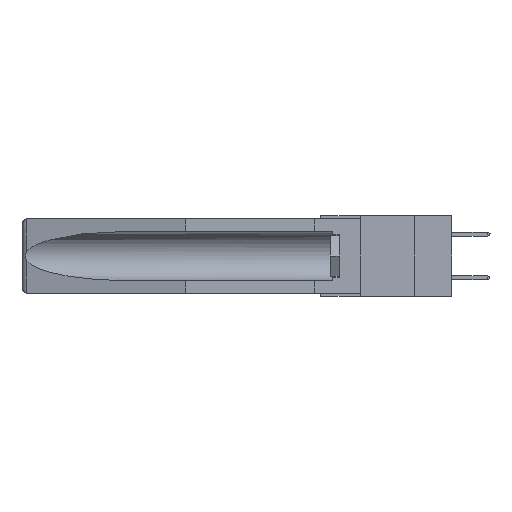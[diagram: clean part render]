
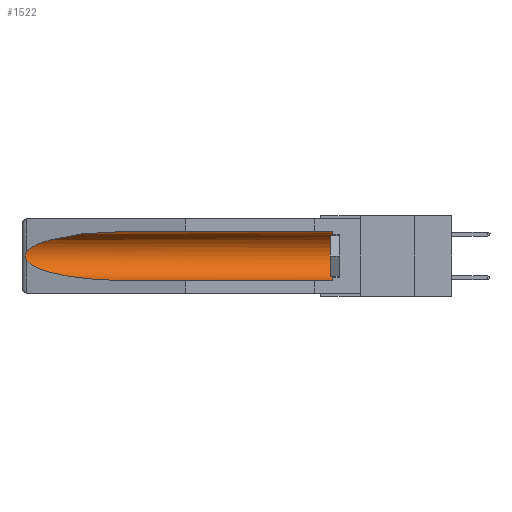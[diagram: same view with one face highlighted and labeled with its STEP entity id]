
A CAD part, left-side view. The second image highlights one B-rep face of the part: STEP entity #1522.
In plain terms, the highlighted cylindrical face has radius 2.857 mm (diameter 5.715 mm), a partial arc.
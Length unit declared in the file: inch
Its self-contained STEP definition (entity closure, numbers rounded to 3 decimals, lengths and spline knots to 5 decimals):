
#142 = ORIENTED_EDGE ( 'NONE', *, *, #10749, .T. ) ;
#1078 = VECTOR ( 'NONE', #8285, 39.37008 ) ;
#1216 = EDGE_CURVE ( 'NONE', #16953, #12645, #14009, .T. ) ;
#1220 = CARTESIAN_POINT ( 'NONE',  ( 0.155, 1.07973, -0.059 ) ) ;
#1522 = ADVANCED_FACE ( 'NONE', ( #5044 ), #20170, .F. ) ;
#1632 = AXIS2_PLACEMENT_3D ( 'NONE', #15619, #21819, #4043 ) ;
#2681 = DIRECTION ( 'NONE',  ( 0., 0., 1. ) ) ;
#3003 = CARTESIAN_POINT ( 'NONE',  ( 0.155, 0.126, -0.284 ) ) ;
#4043 = DIRECTION ( 'NONE',  ( 0., 0., 1. ) ) ;
#4476 = EDGE_CURVE ( 'NONE', #18715, #13065, #6546, .T. ) ;
#5044 = FACE_OUTER_BOUND ( 'NONE', #6459, .T. ) ;
#5306 = CARTESIAN_POINT ( 'NONE',  ( 0.26537, 1.52718, -0.19328 ) ) ;
#5474 = CARTESIAN_POINT ( 'NONE',  ( 0.26597, 1.52961, -0.15275 ) ) ;
#5706 = CARTESIAN_POINT ( 'NONE',  ( 0.155, 1.07973, -0.284 ) ) ;
#6459 = EDGE_LOOP ( 'NONE', ( #12340, #19681, #142, #18638, #24226, #20759 ) ) ;
#6535 = CARTESIAN_POINT ( 'NONE',  ( 0.25451, 1.48313, -0.24835 ) ) ;
#6546 = B_SPLINE_CURVE_WITH_KNOTS ( 'NONE', 3,
 ( #11331, #5474, #15243, #9100, #11079, #10993, #11171, #7032, #9007, #5306 ),
 .UNSPECIFIED., .F., .F.,
 ( 4, 2, 2, 2, 4 ),
 ( 0., 0.00029, 0.00058, 0.00087, 0.00117 ),
 .UNSPECIFIED. ) ;
#7032 = CARTESIAN_POINT ( 'NONE',  ( 0.26655, 1.53094, -0.18657 ) ) ;
#7169 = CARTESIAN_POINT ( 'NONE',  ( 0.26537, 1.52718, -0.14972 ) ) ;
#8103 = CARTESIAN_POINT ( 'NONE',  ( 0.26537, 1.52718, -0.19328 ) ) ;
#8140 = CARTESIAN_POINT ( 'NONE',  ( 0.155, 1.07973, -0.059 ) ) ;
#8285 = DIRECTION ( 'NONE',  ( 0., 1., 0. ) ) ;
#9007 = CARTESIAN_POINT ( 'NONE',  ( 0.26597, 1.5296, -0.19026 ) ) ;
#9100 = CARTESIAN_POINT ( 'NONE',  ( 0.2673, 1.5327, -0.16383 ) ) ;
#10027 =( BOUNDED_CURVE ( )  B_SPLINE_CURVE ( 3, ( #1220, #16964, #22873, #7169 ),
 .UNSPECIFIED., .F., .T. ) 
 B_SPLINE_CURVE_WITH_KNOTS ( ( 4, 4 ),
 ( 4.71239, 6.08839 ),
 .UNSPECIFIED. ) 
 CURVE ( )  GEOMETRIC_REPRESENTATION_ITEM ( )  RATIONAL_B_SPLINE_CURVE ( ( 1., 0.848, 0.848, 1. ) ) 
 REPRESENTATION_ITEM ( '' )  );
#10487 = EDGE_CURVE ( 'NONE', #16953, #22520, #19996, .T. ) ;
#10582 = CARTESIAN_POINT ( 'NONE',  ( 0.155, -0.30754, -0.059 ) ) ;
#10749 = EDGE_CURVE ( 'NONE', #13065, #22520, #17655, .T. ) ;
#10839 = CARTESIAN_POINT ( 'NONE',  ( 0.26537, 1.52718, -0.14972 ) ) ;
#10993 = CARTESIAN_POINT ( 'NONE',  ( 0.2675, 1.53308, -0.17534 ) ) ;
#11079 = CARTESIAN_POINT ( 'NONE',  ( 0.2675, 1.53308, -0.16763 ) ) ;
#11171 = CARTESIAN_POINT ( 'NONE',  ( 0.2673, 1.53269, -0.17917 ) ) ;
#11331 = CARTESIAN_POINT ( 'NONE',  ( 0.26537, 1.52718, -0.14972 ) ) ;
#12340 = ORIENTED_EDGE ( 'NONE', *, *, #14920, .T. ) ;
#12479 = CARTESIAN_POINT ( 'NONE',  ( 0.155, 1.07973, -0.284 ) ) ;
#12645 = VERTEX_POINT ( 'NONE', #22350 ) ;
#13065 = VERTEX_POINT ( 'NONE', #8103 ) ;
#13514 = VECTOR ( 'NONE', #15361, 39.37008 ) ;
#14009 = CIRCLE ( 'NONE', #1632, 0.1125 ) ;
#14920 = EDGE_CURVE ( 'NONE', #17722, #18715, #10027, .T. ) ;
#14989 = LINE ( 'NONE', #10582, #1078 ) ;
#15243 = CARTESIAN_POINT ( 'NONE',  ( 0.26654, 1.53092, -0.15636 ) ) ;
#15361 = DIRECTION ( 'NONE',  ( 0., 1., 0. ) ) ;
#15539 = CARTESIAN_POINT ( 'NONE',  ( 0.155, -0.30754, -0.284 ) ) ;
#15619 = CARTESIAN_POINT ( 'NONE',  ( 0.155, 0.126, -0.1715 ) ) ;
#16953 = VERTEX_POINT ( 'NONE', #3003 ) ;
#16964 = CARTESIAN_POINT ( 'NONE',  ( 0.21114, 1.30732, -0.059 ) ) ;
#17655 =( BOUNDED_CURVE ( )  B_SPLINE_CURVE ( 3, ( #22164, #6535, #20332, #12479 ),
 .UNSPECIFIED., .F., .F. ) 
 B_SPLINE_CURVE_WITH_KNOTS ( ( 4, 4 ),
 ( 0.1948, 1.5708 ),
 .UNSPECIFIED. ) 
 CURVE ( )  GEOMETRIC_REPRESENTATION_ITEM ( )  RATIONAL_B_SPLINE_CURVE ( ( 1., 0.848, 0.848, 1. ) ) 
 REPRESENTATION_ITEM ( '' )  );
#17722 = VERTEX_POINT ( 'NONE', #8140 ) ;
#18638 = ORIENTED_EDGE ( 'NONE', *, *, #10487, .F. ) ;
#18701 = EDGE_CURVE ( 'NONE', #12645, #17722, #14989, .T. ) ;
#18715 = VERTEX_POINT ( 'NONE', #10839 ) ;
#19681 = ORIENTED_EDGE ( 'NONE', *, *, #4476, .T. ) ;
#19958 = CARTESIAN_POINT ( 'NONE',  ( 0.155, -0.30754, -0.1715 ) ) ;
#19996 = LINE ( 'NONE', #15539, #13514 ) ;
#20046 = DIRECTION ( 'NONE',  ( 0., 1., 0. ) ) ;
#20170 = CYLINDRICAL_SURFACE ( 'NONE', #21342, 0.1125 ) ;
#20332 = CARTESIAN_POINT ( 'NONE',  ( 0.21114, 1.30732, -0.284 ) ) ;
#20759 = ORIENTED_EDGE ( 'NONE', *, *, #18701, .T. ) ;
#21342 = AXIS2_PLACEMENT_3D ( 'NONE', #19958, #20046, #2681 ) ;
#21819 = DIRECTION ( 'NONE',  ( 0., -1., 0. ) ) ;
#22164 = CARTESIAN_POINT ( 'NONE',  ( 0.26537, 1.52718, -0.19328 ) ) ;
#22350 = CARTESIAN_POINT ( 'NONE',  ( 0.155, 0.126, -0.059 ) ) ;
#22520 = VERTEX_POINT ( 'NONE', #5706 ) ;
#22873 = CARTESIAN_POINT ( 'NONE',  ( 0.25451, 1.48313, -0.09465 ) ) ;
#24226 = ORIENTED_EDGE ( 'NONE', *, *, #1216, .T. ) ;
